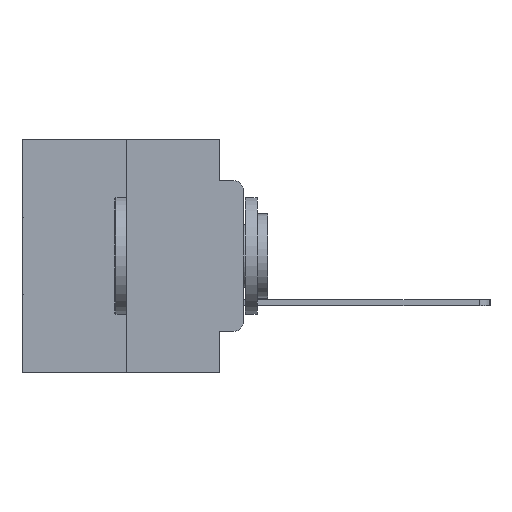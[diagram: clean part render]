
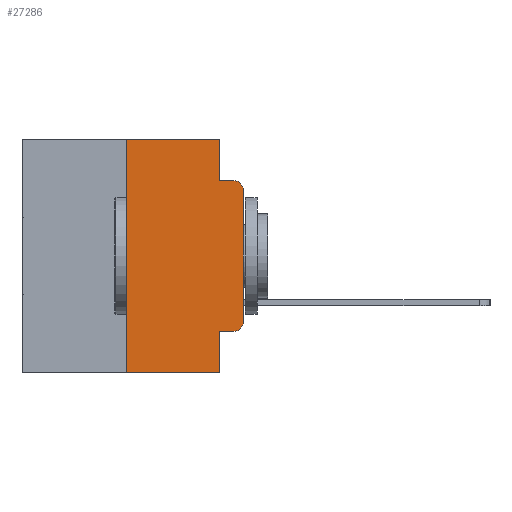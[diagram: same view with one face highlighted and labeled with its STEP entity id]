
A CAD part, left-side view. The second image highlights one B-rep face of the part: STEP entity #27286.
In plain terms, the highlighted planar face has unit normal (-1, 0, 0).
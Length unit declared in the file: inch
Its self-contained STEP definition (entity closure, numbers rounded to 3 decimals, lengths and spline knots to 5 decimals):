
#15 = EDGE_CURVE ( 'NONE', #16805, #26729, #28271, .T. ) ;
#375 = EDGE_CURVE ( 'NONE', #17637, #20577, #20850, .T. ) ;
#940 = ORIENTED_EDGE ( 'NONE', *, *, #12532, .T. ) ;
#1588 = VECTOR ( 'NONE', #6221, 39.37008 ) ;
#1611 = DIRECTION ( 'NONE',  ( 0., -1., 0. ) ) ;
#1958 = VERTEX_POINT ( 'NONE', #13447 ) ;
#1992 = EDGE_CURVE ( 'NONE', #17637, #28444, #13516, .T. ) ;
#2087 = DIRECTION ( 'NONE',  ( 0., 0., -1. ) ) ;
#2397 = ORIENTED_EDGE ( 'NONE', *, *, #8064, .F. ) ;
#2879 = CARTESIAN_POINT ( 'NONE',  ( 0., 0.473, 0. ) ) ;
#2985 = DIRECTION ( 'NONE',  ( 0., 0., 1. ) ) ;
#3529 = EDGE_CURVE ( 'NONE', #1958, #16805, #26792, .T. ) ;
#3858 = ORIENTED_EDGE ( 'NONE', *, *, #3529, .F. ) ;
#4484 = LINE ( 'NONE', #24017, #15627 ) ;
#5314 = ORIENTED_EDGE ( 'NONE', *, *, #26288, .T. ) ;
#5651 = CARTESIAN_POINT ( 'NONE',  ( 0., 0.051, -0.5 ) ) ;
#5699 = CARTESIAN_POINT ( 'NONE',  ( 0., 0.051, -0.4115 ) ) ;
#6211 = CARTESIAN_POINT ( 'NONE',  ( 0., 0.051, -0.0885 ) ) ;
#6221 = DIRECTION ( 'NONE',  ( 0., 0., -1. ) ) ;
#6878 = DIRECTION ( 'NONE',  ( 0., 0., 1. ) ) ;
#7006 = ORIENTED_EDGE ( 'NONE', *, *, #11025, .F. ) ;
#7294 = VECTOR ( 'NONE', #2985, 39.37008 ) ;
#7517 = CARTESIAN_POINT ( 'NONE',  ( 0., 0.051, -0.4115 ) ) ;
#8019 = PLANE ( 'NONE',  #23764 ) ;
#8064 = EDGE_CURVE ( 'NONE', #26729, #28596, #4484, .T. ) ;
#8136 = LINE ( 'NONE', #6211, #18556 ) ;
#8409 = ORIENTED_EDGE ( 'NONE', *, *, #15, .F. ) ;
#8954 = CARTESIAN_POINT ( 'NONE',  ( 0., 0., -0.1085 ) ) ;
#9248 = CARTESIAN_POINT ( 'NONE',  ( 0., 0.25, 0. ) ) ;
#9777 = CIRCLE ( 'NONE', #16886, 0.02 ) ;
#9783 = CARTESIAN_POINT ( 'NONE',  ( 0., 0.473, -0.5 ) ) ;
#9809 = ORIENTED_EDGE ( 'NONE', *, *, #11411, .T. ) ;
#10273 = DIRECTION ( 'NONE',  ( 0., -1., 0. ) ) ;
#11025 = EDGE_CURVE ( 'NONE', #28596, #25505, #8136, .T. ) ;
#11411 = EDGE_CURVE ( 'NONE', #1958, #28444, #27007, .T. ) ;
#11529 = ORIENTED_EDGE ( 'NONE', *, *, #17011, .T. ) ;
#11566 = DIRECTION ( 'NONE',  ( -1., 0., 0. ) ) ;
#12103 = VERTEX_POINT ( 'NONE', #14415 ) ;
#12252 = CARTESIAN_POINT ( 'NONE',  ( 0., 0.02, -0.4115 ) ) ;
#12532 = EDGE_CURVE ( 'NONE', #13346, #25505, #9777, .T. ) ;
#13179 = AXIS2_PLACEMENT_3D ( 'NONE', #28512, #15512, #2087 ) ;
#13270 = CARTESIAN_POINT ( 'NONE',  ( 0., 0.25, 0. ) ) ;
#13346 = VERTEX_POINT ( 'NONE', #8954 ) ;
#13447 = CARTESIAN_POINT ( 'NONE',  ( 0., 0.25, -0.5 ) ) ;
#13516 = LINE ( 'NONE', #18376, #1588 ) ;
#13898 = LINE ( 'NONE', #14149, #7294 ) ;
#14149 = CARTESIAN_POINT ( 'NONE',  ( 0., 0., 0. ) ) ;
#14415 = CARTESIAN_POINT ( 'NONE',  ( 0., 0., -0.3915 ) ) ;
#14714 = DIRECTION ( 'NONE',  ( 0., 0., -1. ) ) ;
#15512 = DIRECTION ( 'NONE',  ( -1., 0., 0. ) ) ;
#15627 = VECTOR ( 'NONE', #26132, 39.37008 ) ;
#15727 = ORIENTED_EDGE ( 'NONE', *, *, #1992, .F. ) ;
#16772 = VECTOR ( 'NONE', #10273, 39.37008 ) ;
#16805 = VERTEX_POINT ( 'NONE', #13270 ) ;
#16873 = CARTESIAN_POINT ( 'NONE',  ( 0., 0.473, 0. ) ) ;
#16886 = AXIS2_PLACEMENT_3D ( 'NONE', #24742, #11566, #26894 ) ;
#17011 = EDGE_CURVE ( 'NONE', #12103, #13346, #13898, .T. ) ;
#17637 = VERTEX_POINT ( 'NONE', #7517 ) ;
#17755 = CIRCLE ( 'NONE', #13179, 0.02 ) ;
#18376 = CARTESIAN_POINT ( 'NONE',  ( 0., 0.051, 0. ) ) ;
#18556 = VECTOR ( 'NONE', #1611, 39.37008 ) ;
#19248 = CARTESIAN_POINT ( 'NONE',  ( 0., 0.051, 0. ) ) ;
#19371 = CARTESIAN_POINT ( 'NONE',  ( 0., 0.051, -0.0885 ) ) ;
#19376 = FACE_OUTER_BOUND ( 'NONE', #21551, .T. ) ;
#20577 = VERTEX_POINT ( 'NONE', #12252 ) ;
#20850 = LINE ( 'NONE', #5699, #25259 ) ;
#20908 = DIRECTION ( 'NONE',  ( 0., -1., 0. ) ) ;
#21038 = VECTOR ( 'NONE', #6878, 39.37008 ) ;
#21551 = EDGE_LOOP ( 'NONE', ( #11529, #940, #7006, #2397, #8409, #3858, #9809, #15727, #27967, #5314 ) ) ;
#23764 = AXIS2_PLACEMENT_3D ( 'NONE', #16873, #27767, #14714 ) ;
#24017 = CARTESIAN_POINT ( 'NONE',  ( 0., 0.051, 0. ) ) ;
#24742 = CARTESIAN_POINT ( 'NONE',  ( 0., 0.02, -0.1085 ) ) ;
#25259 = VECTOR ( 'NONE', #25797, 39.37008 ) ;
#25505 = VERTEX_POINT ( 'NONE', #27820 ) ;
#25661 = VECTOR ( 'NONE', #20908, 39.37008 ) ;
#25797 = DIRECTION ( 'NONE',  ( 0., -1., 0. ) ) ;
#26132 = DIRECTION ( 'NONE',  ( 0., 0., -1. ) ) ;
#26288 = EDGE_CURVE ( 'NONE', #20577, #12103, #17755, .T. ) ;
#26729 = VERTEX_POINT ( 'NONE', #19248 ) ;
#26792 = LINE ( 'NONE', #9248, #21038 ) ;
#26894 = DIRECTION ( 'NONE',  ( 0., 0., -1. ) ) ;
#27007 = LINE ( 'NONE', #9783, #25661 ) ;
#27286 = ADVANCED_FACE ( 'NONE', ( #19376 ), #8019, .F. ) ;
#27767 = DIRECTION ( 'NONE',  ( 1., 0., 0. ) ) ;
#27820 = CARTESIAN_POINT ( 'NONE',  ( 0., 0.02, -0.0885 ) ) ;
#27967 = ORIENTED_EDGE ( 'NONE', *, *, #375, .T. ) ;
#28271 = LINE ( 'NONE', #2879, #16772 ) ;
#28444 = VERTEX_POINT ( 'NONE', #5651 ) ;
#28512 = CARTESIAN_POINT ( 'NONE',  ( 0., 0.02, -0.3915 ) ) ;
#28596 = VERTEX_POINT ( 'NONE', #19371 ) ;
